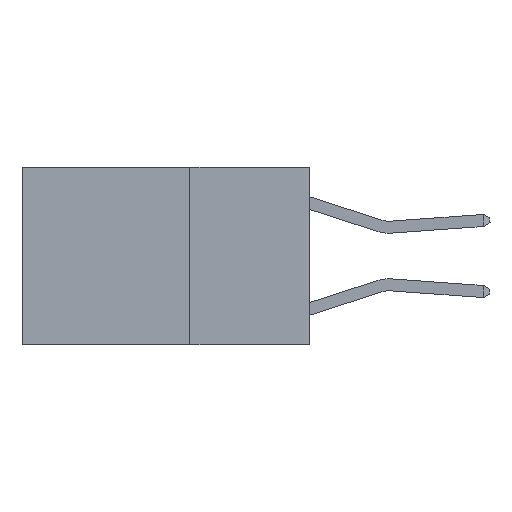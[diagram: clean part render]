
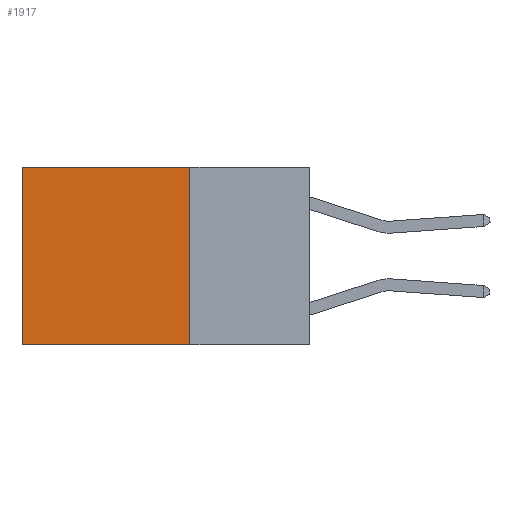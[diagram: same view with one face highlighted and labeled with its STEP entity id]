
A CAD part, left-side view. The second image highlights one B-rep face of the part: STEP entity #1917.
In plain terms, the highlighted planar face has unit normal (-1, 0, 0).
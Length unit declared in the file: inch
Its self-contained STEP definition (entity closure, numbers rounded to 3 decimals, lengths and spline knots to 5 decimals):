
#2 = VECTOR ( 'NONE', #3526, 39.37008 ) ;
#793 = EDGE_LOOP ( 'NONE', ( #5844, #1837, #4100, #8540 ) ) ;
#844 = PLANE ( 'NONE',  #7867 ) ;
#1179 = LINE ( 'NONE', #1909, #2896 ) ;
#1790 = CARTESIAN_POINT ( 'NONE',  ( 0.2625, 0.6, -0.37 ) ) ;
#1837 = ORIENTED_EDGE ( 'NONE', *, *, #6520, .F. ) ;
#1909 = CARTESIAN_POINT ( 'NONE',  ( 0.2625, 0.25, 0. ) ) ;
#1917 = ADVANCED_FACE ( 'NONE', ( #10091 ), #844, .F. ) ;
#2597 = LINE ( 'NONE', #9861, #9173 ) ;
#2742 = DIRECTION ( 'NONE',  ( 0., 0., -1. ) ) ;
#2769 = EDGE_CURVE ( 'NONE', #8555, #7706, #2597, .T. ) ;
#2896 = VECTOR ( 'NONE', #2742, 39.37008 ) ;
#3239 = DIRECTION ( 'NONE',  ( 1., 0., 0. ) ) ;
#3526 = DIRECTION ( 'NONE',  ( 0., 0., -1. ) ) ;
#3648 = CARTESIAN_POINT ( 'NONE',  ( 0.2625, 0.25, -0.37 ) ) ;
#4100 = ORIENTED_EDGE ( 'NONE', *, *, #9008, .F. ) ;
#4436 = CARTESIAN_POINT ( 'NONE',  ( 0.2625, 0.6, 0. ) ) ;
#4663 = VERTEX_POINT ( 'NONE', #1790 ) ;
#4890 = DIRECTION ( 'NONE',  ( 0., 0., -1. ) ) ;
#5156 = VECTOR ( 'NONE', #9958, 39.37008 ) ;
#5158 = CARTESIAN_POINT ( 'NONE',  ( 0.2625, 0.25, 0. ) ) ;
#5844 = ORIENTED_EDGE ( 'NONE', *, *, #7068, .T. ) ;
#6520 = EDGE_CURVE ( 'NONE', #7593, #4663, #7504, .T. ) ;
#6967 = CARTESIAN_POINT ( 'NONE',  ( 0.2625, 0.25, 0. ) ) ;
#7068 = EDGE_CURVE ( 'NONE', #7706, #4663, #8587, .T. ) ;
#7504 = LINE ( 'NONE', #3648, #5156 ) ;
#7593 = VERTEX_POINT ( 'NONE', #8200 ) ;
#7706 = VERTEX_POINT ( 'NONE', #4436 ) ;
#7867 = AXIS2_PLACEMENT_3D ( 'NONE', #5158, #3239, #4890 ) ;
#8200 = CARTESIAN_POINT ( 'NONE',  ( 0.2625, 0.25, -0.37 ) ) ;
#8260 = DIRECTION ( 'NONE',  ( 0., 1., 0. ) ) ;
#8540 = ORIENTED_EDGE ( 'NONE', *, *, #2769, .T. ) ;
#8555 = VERTEX_POINT ( 'NONE', #6967 ) ;
#8587 = LINE ( 'NONE', #9069, #2 ) ;
#9008 = EDGE_CURVE ( 'NONE', #8555, #7593, #1179, .T. ) ;
#9069 = CARTESIAN_POINT ( 'NONE',  ( 0.2625, 0.6, 0. ) ) ;
#9173 = VECTOR ( 'NONE', #8260, 39.37008 ) ;
#9861 = CARTESIAN_POINT ( 'NONE',  ( 0.2625, 0.25, 0. ) ) ;
#9958 = DIRECTION ( 'NONE',  ( 0., 1., 0. ) ) ;
#10091 = FACE_OUTER_BOUND ( 'NONE', #793, .T. ) ;
